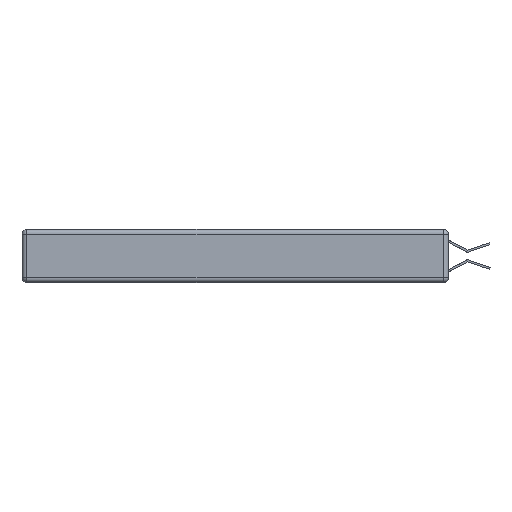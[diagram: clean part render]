
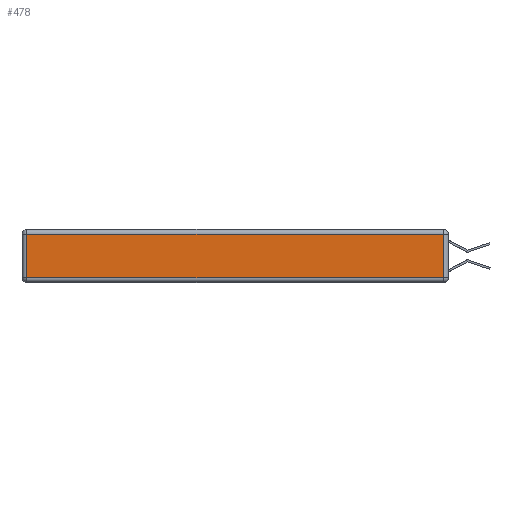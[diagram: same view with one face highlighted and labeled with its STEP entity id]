
A CAD part, left-side view. The second image highlights one B-rep face of the part: STEP entity #478.
In plain terms, the highlighted planar face has unit normal (-1, 0, 0).
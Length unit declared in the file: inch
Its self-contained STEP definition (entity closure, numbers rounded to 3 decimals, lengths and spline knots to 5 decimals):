
#274 = ORIENTED_EDGE ( 'NONE', *, *, #11687, .T. ) ;
#325 = VECTOR ( 'NONE', #15119, 39.37008 ) ;
#478 = ADVANCED_FACE ( 'NONE', ( #5453 ), #4302, .T. ) ;
#534 = DIRECTION ( 'NONE',  ( -1., 0., 0. ) ) ;
#1165 = CARTESIAN_POINT ( 'NONE',  ( 0., 2.72, -0.343 ) ) ;
#1860 = VERTEX_POINT ( 'NONE', #12242 ) ;
#2214 = EDGE_CURVE ( 'NONE', #1860, #10791, #3071, .T. ) ;
#2850 = DIRECTION ( 'NONE',  ( 0., 0., 1. ) ) ;
#3071 = LINE ( 'NONE', #4139, #7029 ) ;
#3198 = CARTESIAN_POINT ( 'NONE',  ( 0., 0.03, -0.03 ) ) ;
#4139 = CARTESIAN_POINT ( 'NONE',  ( 0., 0.03, -0.343 ) ) ;
#4302 = PLANE ( 'NONE',  #15761 ) ;
#4368 = DIRECTION ( 'NONE',  ( 0., 0., 1. ) ) ;
#4730 = EDGE_CURVE ( 'NONE', #15411, #1860, #9664, .T. ) ;
#4773 = DIRECTION ( 'NONE',  ( 0., 0., -1. ) ) ;
#5453 = FACE_OUTER_BOUND ( 'NONE', #7218, .T. ) ;
#5617 = CARTESIAN_POINT ( 'NONE',  ( 0., 0., -0.343 ) ) ;
#6512 = CARTESIAN_POINT ( 'NONE',  ( 0., 2.75, -0.03 ) ) ;
#6705 = ORIENTED_EDGE ( 'NONE', *, *, #10038, .T. ) ;
#7029 = VECTOR ( 'NONE', #4368, 39.37008 ) ;
#7218 = EDGE_LOOP ( 'NONE', ( #11225, #8315, #6705, #274 ) ) ;
#7396 = VECTOR ( 'NONE', #11510, 39.37008 ) ;
#7593 = LINE ( 'NONE', #6512, #7396 ) ;
#7612 = CARTESIAN_POINT ( 'NONE',  ( 0., 2.72, -0.03 ) ) ;
#8315 = ORIENTED_EDGE ( 'NONE', *, *, #2214, .T. ) ;
#9664 = LINE ( 'NONE', #13600, #325 ) ;
#10038 = EDGE_CURVE ( 'NONE', #10791, #11251, #7593, .T. ) ;
#10791 = VERTEX_POINT ( 'NONE', #3198 ) ;
#11225 = ORIENTED_EDGE ( 'NONE', *, *, #4730, .T. ) ;
#11251 = VERTEX_POINT ( 'NONE', #7612 ) ;
#11510 = DIRECTION ( 'NONE',  ( 0., 1., 0. ) ) ;
#11687 = EDGE_CURVE ( 'NONE', #11251, #15411, #14897, .T. ) ;
#12242 = CARTESIAN_POINT ( 'NONE',  ( 0., 0.03, -0.313 ) ) ;
#13600 = CARTESIAN_POINT ( 'NONE',  ( 0., 0., -0.313 ) ) ;
#14897 = LINE ( 'NONE', #1165, #15275 ) ;
#15119 = DIRECTION ( 'NONE',  ( 0., -1., 0. ) ) ;
#15121 = CARTESIAN_POINT ( 'NONE',  ( 0., 2.72, -0.313 ) ) ;
#15275 = VECTOR ( 'NONE', #4773, 39.37008 ) ;
#15411 = VERTEX_POINT ( 'NONE', #15121 ) ;
#15761 = AXIS2_PLACEMENT_3D ( 'NONE', #5617, #534, #2850 ) ;
